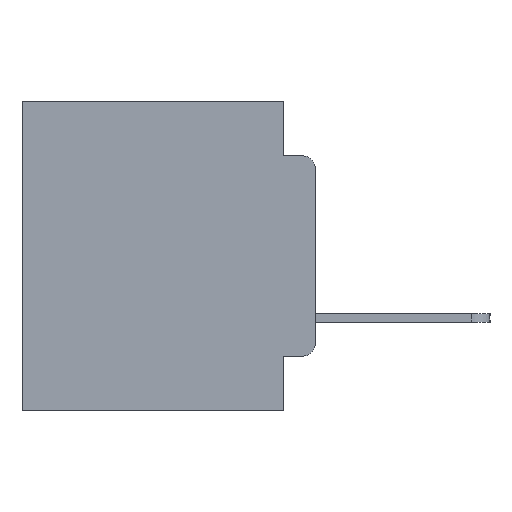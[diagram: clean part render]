
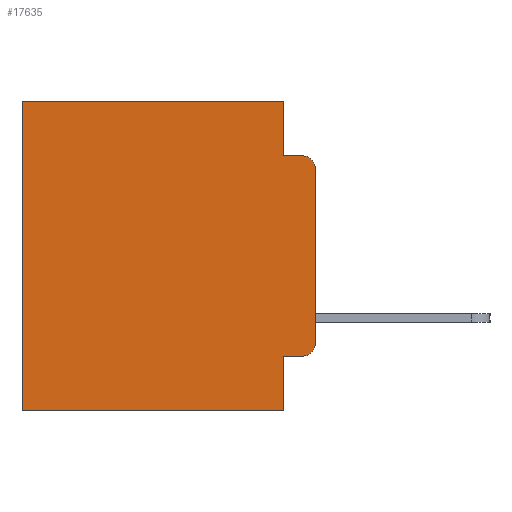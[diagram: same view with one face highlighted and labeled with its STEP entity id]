
A CAD part, left-side view. The second image highlights one B-rep face of the part: STEP entity #17635.
In plain terms, the highlighted planar face has unit normal (-1, 0, 0).
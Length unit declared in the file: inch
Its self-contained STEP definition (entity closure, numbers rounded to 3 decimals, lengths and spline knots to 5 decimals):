
#99 = FACE_OUTER_BOUND ( 'NONE', #16708, .T. ) ;
#120 = DIRECTION ( 'NONE',  ( -1., 0., 0. ) ) ;
#217 = CARTESIAN_POINT ( 'NONE',  ( 0.298, 0.051, -0.5 ) ) ;
#573 = CARTESIAN_POINT ( 'NONE',  ( 0.298, 0.02, -0.1085 ) ) ;
#611 = EDGE_CURVE ( 'NONE', #22777, #15905, #21315, .T. ) ;
#1209 = ORIENTED_EDGE ( 'NONE', *, *, #2030, .F. ) ;
#1240 = CIRCLE ( 'NONE', #20166, 0.02 ) ;
#2030 = EDGE_CURVE ( 'NONE', #11846, #20841, #5857, .T. ) ;
#2101 = VERTEX_POINT ( 'NONE', #19828 ) ;
#2148 = ORIENTED_EDGE ( 'NONE', *, *, #7474, .F. ) ;
#2674 = DIRECTION ( 'NONE',  ( 0., 0., -1. ) ) ;
#2744 = CARTESIAN_POINT ( 'NONE',  ( 0.298, 0.051, -0.0885 ) ) ;
#2833 = VERTEX_POINT ( 'NONE', #4945 ) ;
#2853 = VERTEX_POINT ( 'NONE', #12065 ) ;
#3030 = CARTESIAN_POINT ( 'NONE',  ( 0.298, 0.473, 0. ) ) ;
#4641 = CIRCLE ( 'NONE', #11271, 0.02 ) ;
#4714 = PLANE ( 'NONE',  #24501 ) ;
#4945 = CARTESIAN_POINT ( 'NONE',  ( 0.298, 0.051, 0. ) ) ;
#5184 = LINE ( 'NONE', #25709, #10639 ) ;
#5402 = CARTESIAN_POINT ( 'NONE',  ( 0.298, 0.473, -0.5 ) ) ;
#5857 = LINE ( 'NONE', #20754, #6489 ) ;
#6489 = VECTOR ( 'NONE', #20799, 39.37008 ) ;
#6766 = DIRECTION ( 'NONE',  ( 1., 0., 0. ) ) ;
#7474 = EDGE_CURVE ( 'NONE', #2853, #2101, #10267, .T. ) ;
#7525 = EDGE_CURVE ( 'NONE', #20841, #15905, #14374, .T. ) ;
#7655 = CARTESIAN_POINT ( 'NONE',  ( 0.298, 0., -0.3915 ) ) ;
#8583 = ORIENTED_EDGE ( 'NONE', *, *, #611, .T. ) ;
#8760 = DIRECTION ( 'NONE',  ( 0., 0., -1. ) ) ;
#9045 = DIRECTION ( 'NONE',  ( 0., 1., 0. ) ) ;
#9609 = ORIENTED_EDGE ( 'NONE', *, *, #20157, .T. ) ;
#9621 = VECTOR ( 'NONE', #18914, 39.37008 ) ;
#9708 = CARTESIAN_POINT ( 'NONE',  ( 0.298, 0.02, -0.4115 ) ) ;
#9842 = LINE ( 'NONE', #10954, #24356 ) ;
#10240 = EDGE_CURVE ( 'NONE', #2833, #2853, #9842, .T. ) ;
#10267 = LINE ( 'NONE', #2744, #9621 ) ;
#10620 = ORIENTED_EDGE ( 'NONE', *, *, #17471, .T. ) ;
#10639 = VECTOR ( 'NONE', #20064, 39.37008 ) ;
#10685 = VECTOR ( 'NONE', #10940, 39.37008 ) ;
#10814 = DIRECTION ( 'NONE',  ( 0., 1., 0. ) ) ;
#10940 = DIRECTION ( 'NONE',  ( 0., 0., -1. ) ) ;
#10954 = CARTESIAN_POINT ( 'NONE',  ( 0.298, 0.051, 0. ) ) ;
#11191 = CARTESIAN_POINT ( 'NONE',  ( 0.298, 0.051, -0.4115 ) ) ;
#11271 = AXIS2_PLACEMENT_3D ( 'NONE', #12375, #120, #14439 ) ;
#11846 = VERTEX_POINT ( 'NONE', #11191 ) ;
#12051 = CARTESIAN_POINT ( 'NONE',  ( 0.298, 0., -0.1085 ) ) ;
#12065 = CARTESIAN_POINT ( 'NONE',  ( 0.298, 0.051, -0.0885 ) ) ;
#12375 = CARTESIAN_POINT ( 'NONE',  ( 0.298, 0.02, -0.3915 ) ) ;
#12577 = ORIENTED_EDGE ( 'NONE', *, *, #10240, .F. ) ;
#12984 = DIRECTION ( 'NONE',  ( 0., 0., -1. ) ) ;
#14374 = LINE ( 'NONE', #22940, #24156 ) ;
#14439 = DIRECTION ( 'NONE',  ( 0., 0., -1. ) ) ;
#14773 = VERTEX_POINT ( 'NONE', #12051 ) ;
#14853 = DIRECTION ( 'NONE',  ( -1., 0., 0. ) ) ;
#15638 = EDGE_CURVE ( 'NONE', #14773, #2101, #1240, .T. ) ;
#15905 = VERTEX_POINT ( 'NONE', #5402 ) ;
#16035 = LINE ( 'NONE', #18926, #10685 ) ;
#16092 = VECTOR ( 'NONE', #8760, 39.37008 ) ;
#16694 = ORIENTED_EDGE ( 'NONE', *, *, #20924, .T. ) ;
#16708 = EDGE_LOOP ( 'NONE', ( #25071, #25154, #2148, #12577, #16694, #8583, #22563, #1209, #9609, #10620 ) ) ;
#16874 = CARTESIAN_POINT ( 'NONE',  ( 0.298, 0., 0. ) ) ;
#17471 = EDGE_CURVE ( 'NONE', #21796, #21198, #4641, .T. ) ;
#17635 = ADVANCED_FACE ( 'NONE', ( #99 ), #4714, .F. ) ;
#18313 = EDGE_CURVE ( 'NONE', #14773, #21198, #16035, .T. ) ;
#18914 = DIRECTION ( 'NONE',  ( 0., -1., 0. ) ) ;
#18926 = CARTESIAN_POINT ( 'NONE',  ( 0.298, 0., 0. ) ) ;
#19828 = CARTESIAN_POINT ( 'NONE',  ( 0.298, 0.02, -0.0885 ) ) ;
#20064 = DIRECTION ( 'NONE',  ( 0., -1., 0. ) ) ;
#20157 = EDGE_CURVE ( 'NONE', #11846, #21796, #5184, .T. ) ;
#20166 = AXIS2_PLACEMENT_3D ( 'NONE', #573, #14853, #2674 ) ;
#20754 = CARTESIAN_POINT ( 'NONE',  ( 0.298, 0.051, 0. ) ) ;
#20799 = DIRECTION ( 'NONE',  ( 0., 0., -1. ) ) ;
#20831 = DIRECTION ( 'NONE',  ( 0., 0., -1. ) ) ;
#20841 = VERTEX_POINT ( 'NONE', #217 ) ;
#20924 = EDGE_CURVE ( 'NONE', #2833, #22777, #25657, .T. ) ;
#21166 = VECTOR ( 'NONE', #10814, 39.37008 ) ;
#21198 = VERTEX_POINT ( 'NONE', #7655 ) ;
#21315 = LINE ( 'NONE', #3030, #16092 ) ;
#21796 = VERTEX_POINT ( 'NONE', #9708 ) ;
#22367 = CARTESIAN_POINT ( 'NONE',  ( 0.298, 0.473, 0. ) ) ;
#22563 = ORIENTED_EDGE ( 'NONE', *, *, #7525, .F. ) ;
#22653 = CARTESIAN_POINT ( 'NONE',  ( 0.298, 0., 0. ) ) ;
#22777 = VERTEX_POINT ( 'NONE', #22367 ) ;
#22940 = CARTESIAN_POINT ( 'NONE',  ( 0.298, 0., -0.5 ) ) ;
#24156 = VECTOR ( 'NONE', #9045, 39.37008 ) ;
#24356 = VECTOR ( 'NONE', #12984, 39.37008 ) ;
#24501 = AXIS2_PLACEMENT_3D ( 'NONE', #16874, #6766, #20831 ) ;
#25071 = ORIENTED_EDGE ( 'NONE', *, *, #18313, .F. ) ;
#25154 = ORIENTED_EDGE ( 'NONE', *, *, #15638, .T. ) ;
#25657 = LINE ( 'NONE', #22653, #21166 ) ;
#25709 = CARTESIAN_POINT ( 'NONE',  ( 0.298, 0.051, -0.4115 ) ) ;
